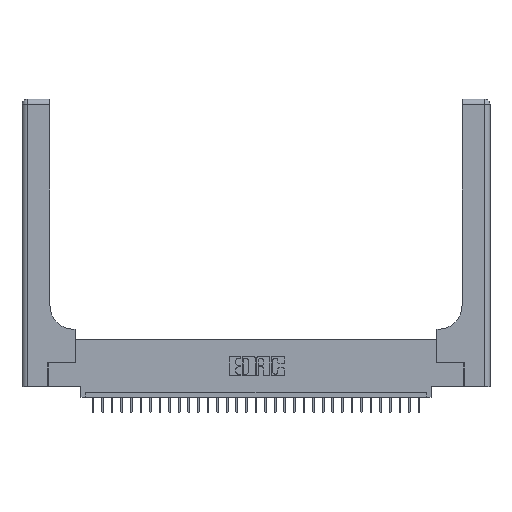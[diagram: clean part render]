
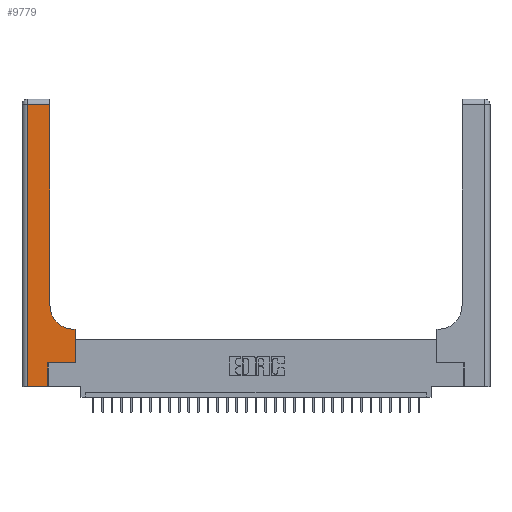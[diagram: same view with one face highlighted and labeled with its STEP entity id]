
A CAD part, top view. The second image highlights one B-rep face of the part: STEP entity #9779.
In plain terms, the highlighted planar face has unit normal (0, 0, 1).
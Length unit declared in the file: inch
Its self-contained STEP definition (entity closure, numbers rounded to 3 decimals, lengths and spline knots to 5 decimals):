
#760 = DIRECTION ( 'NONE',  ( 0., 0., -1. ) ) ;
#1759 = CARTESIAN_POINT ( 'NONE',  ( 0.269, 0., 0.37 ) ) ;
#2497 = EDGE_CURVE ( 'NONE', #25878, #28125, #3560, .T. ) ;
#3380 = DIRECTION ( 'NONE',  ( 1., 0., 0. ) ) ;
#3431 = PLANE ( 'NONE',  #26162 ) ;
#3560 = LINE ( 'NONE', #21032, #20473 ) ;
#4490 = ORIENTED_EDGE ( 'NONE', *, *, #24086, .T. ) ;
#4606 = LINE ( 'NONE', #7687, #12875 ) ;
#5247 = CARTESIAN_POINT ( 'NONE',  ( 0.2915, 0.6, 0.37 ) ) ;
#6234 = EDGE_CURVE ( 'NONE', #20709, #32569, #18675, .T. ) ;
#6378 = ORIENTED_EDGE ( 'NONE', *, *, #18643, .T. ) ;
#6581 = CARTESIAN_POINT ( 'NONE',  ( 0.5585, 0.25, 0.37 ) ) ;
#7687 = CARTESIAN_POINT ( 'NONE',  ( 0.269, 0.25, 0.37 ) ) ;
#7785 = VERTEX_POINT ( 'NONE', #6581 ) ;
#8473 = EDGE_CURVE ( 'NONE', #26330, #15596, #13116, .T. ) ;
#8501 = DIRECTION ( 'NONE',  ( 1., 0., 0. ) ) ;
#9252 = ORIENTED_EDGE ( 'NONE', *, *, #25152, .T. ) ;
#9779 = ADVANCED_FACE ( 'NONE', ( #15066 ), #3431, .F. ) ;
#10390 = VECTOR ( 'NONE', #20392, 39.37008 ) ;
#10437 = DIRECTION ( 'NONE',  ( 0., -1., 0. ) ) ;
#10465 = ORIENTED_EDGE ( 'NONE', *, *, #6234, .T. ) ;
#11018 = CIRCLE ( 'NONE', #17004, 0.25 ) ;
#11073 = CARTESIAN_POINT ( 'NONE',  ( 0.2915, 3., 0.37 ) ) ;
#11108 = CARTESIAN_POINT ( 'NONE',  ( 0., 3., 0.37 ) ) ;
#11149 = CARTESIAN_POINT ( 'NONE',  ( 0.269, 0.25, 0.37 ) ) ;
#12798 = CARTESIAN_POINT ( 'NONE',  ( 0.5585, 0.6, 0.37 ) ) ;
#12875 = VECTOR ( 'NONE', #13069, 39.37008 ) ;
#13069 = DIRECTION ( 'NONE',  ( 1., 0., 0. ) ) ;
#13116 = LINE ( 'NONE', #11073, #15878 ) ;
#13414 = VECTOR ( 'NONE', #31136, 39.37008 ) ;
#13531 = DIRECTION ( 'NONE',  ( -1., 0., 0. ) ) ;
#14015 = EDGE_CURVE ( 'NONE', #28125, #22683, #19514, .T. ) ;
#15066 = FACE_OUTER_BOUND ( 'NONE', #30780, .T. ) ;
#15268 = CARTESIAN_POINT ( 'NONE',  ( 0.06, 0., 0.37 ) ) ;
#15596 = VERTEX_POINT ( 'NONE', #26552 ) ;
#15878 = VECTOR ( 'NONE', #21526, 39.37008 ) ;
#15954 = EDGE_CURVE ( 'NONE', #22683, #7785, #4606, .T. ) ;
#16684 = LINE ( 'NONE', #28368, #10390 ) ;
#17004 = AXIS2_PLACEMENT_3D ( 'NONE', #18557, #18233, #3380 ) ;
#18040 = CARTESIAN_POINT ( 'NONE',  ( 0.06, 3., 0.37 ) ) ;
#18233 = DIRECTION ( 'NONE',  ( 0., 0., -1. ) ) ;
#18300 = ORIENTED_EDGE ( 'NONE', *, *, #14015, .T. ) ;
#18557 = CARTESIAN_POINT ( 'NONE',  ( 0.5415, 0.85, 0.37 ) ) ;
#18643 = EDGE_CURVE ( 'NONE', #15596, #28170, #16684, .T. ) ;
#18675 = LINE ( 'NONE', #5247, #23000 ) ;
#18683 = VECTOR ( 'NONE', #10437, 39.37008 ) ;
#18972 = CARTESIAN_POINT ( 'NONE',  ( 0.269, 0., 0.37 ) ) ;
#19514 = LINE ( 'NONE', #1759, #22315 ) ;
#20392 = DIRECTION ( 'NONE',  ( -1., 0., 0. ) ) ;
#20473 = VECTOR ( 'NONE', #8501, 39.37008 ) ;
#20709 = VERTEX_POINT ( 'NONE', #12798 ) ;
#21032 = CARTESIAN_POINT ( 'NONE',  ( 0., 0., 0.37 ) ) ;
#21171 = CARTESIAN_POINT ( 'NONE',  ( 0.5585, 0.25, 0.37 ) ) ;
#21526 = DIRECTION ( 'NONE',  ( 0., 1., 0. ) ) ;
#22315 = VECTOR ( 'NONE', #29341, 39.37008 ) ;
#22415 = ORIENTED_EDGE ( 'NONE', *, *, #32301, .T. ) ;
#22683 = VERTEX_POINT ( 'NONE', #11149 ) ;
#22859 = LINE ( 'NONE', #21171, #13414 ) ;
#22868 = DIRECTION ( 'NONE',  ( -1., 0., 0. ) ) ;
#23000 = VECTOR ( 'NONE', #22868, 39.37008 ) ;
#23887 = ORIENTED_EDGE ( 'NONE', *, *, #2497, .T. ) ;
#24086 = EDGE_CURVE ( 'NONE', #7785, #20709, #22859, .T. ) ;
#25152 = EDGE_CURVE ( 'NONE', #32569, #26330, #11018, .T. ) ;
#25878 = VERTEX_POINT ( 'NONE', #15268 ) ;
#26162 = AXIS2_PLACEMENT_3D ( 'NONE', #11108, #760, #13531 ) ;
#26277 = CARTESIAN_POINT ( 'NONE',  ( 0.2915, 0.85, 0.37 ) ) ;
#26305 = CARTESIAN_POINT ( 'NONE',  ( 0.5415, 0.6, 0.37 ) ) ;
#26330 = VERTEX_POINT ( 'NONE', #26277 ) ;
#26552 = CARTESIAN_POINT ( 'NONE',  ( 0.2915, 2.94, 0.37 ) ) ;
#27321 = ORIENTED_EDGE ( 'NONE', *, *, #8473, .T. ) ;
#28125 = VERTEX_POINT ( 'NONE', #18972 ) ;
#28170 = VERTEX_POINT ( 'NONE', #29030 ) ;
#28368 = CARTESIAN_POINT ( 'NONE',  ( 0., 2.94, 0.37 ) ) ;
#29030 = CARTESIAN_POINT ( 'NONE',  ( 0.06, 2.94, 0.37 ) ) ;
#29341 = DIRECTION ( 'NONE',  ( 0., 1., 0. ) ) ;
#30161 = LINE ( 'NONE', #18040, #18683 ) ;
#30780 = EDGE_LOOP ( 'NONE', ( #27321, #6378, #22415, #23887, #18300, #31147, #4490, #10465, #9252 ) ) ;
#31136 = DIRECTION ( 'NONE',  ( 0., 1., 0. ) ) ;
#31147 = ORIENTED_EDGE ( 'NONE', *, *, #15954, .T. ) ;
#32301 = EDGE_CURVE ( 'NONE', #28170, #25878, #30161, .T. ) ;
#32569 = VERTEX_POINT ( 'NONE', #26305 ) ;
